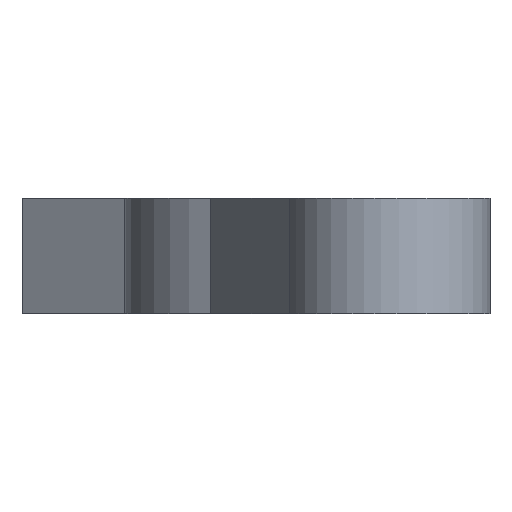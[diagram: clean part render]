
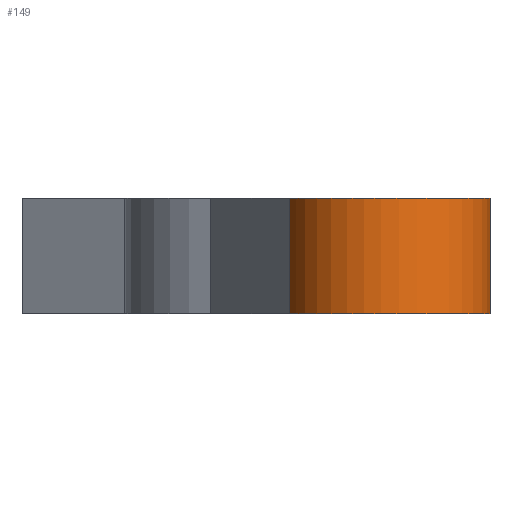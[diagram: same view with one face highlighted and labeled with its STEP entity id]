
A CAD part, left-side view. The second image highlights one B-rep face of the part: STEP entity #149.
In plain terms, the highlighted cylindrical face has radius 4.216 mm (diameter 8.433 mm), a partial arc.
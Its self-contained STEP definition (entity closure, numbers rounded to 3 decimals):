
#3 = VECTOR ( 'NONE', #229, 1000. ) ;
#41 = EDGE_LOOP ( 'NONE', ( #305, #256, #509, #240 ) ) ;
#48 = CIRCLE ( 'NONE', #468, 4.216 ) ;
#68 = DIRECTION ( 'NONE',  ( 1., 0., 0. ) ) ;
#91 = LINE ( 'NONE', #261, #3 ) ;
#96 = LINE ( 'NONE', #133, #669 ) ;
#127 = CARTESIAN_POINT ( 'NONE',  ( 97.778, 23.491, -10.65 ) ) ;
#133 = CARTESIAN_POINT ( 'NONE',  ( 100.156, 15.4, -10.65 ) ) ;
#149 = ADVANCED_FACE ( 'NONE', ( #674 ), #379, .T. ) ;
#167 = DIRECTION ( 'NONE',  ( 0., 0., 1. ) ) ;
#211 = VERTEX_POINT ( 'NONE', #606 ) ;
#222 = CARTESIAN_POINT ( 'NONE',  ( 100.156, 15.4, -10.65 ) ) ;
#229 = DIRECTION ( 'NONE',  ( 0., 0., 1. ) ) ;
#240 = ORIENTED_EDGE ( 'NONE', *, *, #474, .T. ) ;
#256 = ORIENTED_EDGE ( 'NONE', *, *, #407, .F. ) ;
#261 = CARTESIAN_POINT ( 'NONE',  ( 97.778, 23.491, -10.65 ) ) ;
#275 = EDGE_CURVE ( 'NONE', #470, #414, #473, .T. ) ;
#282 = CARTESIAN_POINT ( 'NONE',  ( 97.778, 23.491, -5.9 ) ) ;
#305 = ORIENTED_EDGE ( 'NONE', *, *, #343, .F. ) ;
#323 = DIRECTION ( 'NONE',  ( 0., 0., 1. ) ) ;
#343 = EDGE_CURVE ( 'NONE', #402, #211, #48, .T. ) ;
#379 = CYLINDRICAL_SURFACE ( 'NONE', #582, 4.216 ) ;
#402 = VERTEX_POINT ( 'NONE', #282 ) ;
#407 = EDGE_CURVE ( 'NONE', #470, #402, #91, .T. ) ;
#414 = VERTEX_POINT ( 'NONE', #222 ) ;
#430 = DIRECTION ( 'NONE',  ( 1., 0., 0. ) ) ;
#435 = DIRECTION ( 'NONE',  ( 0., 0., 1. ) ) ;
#437 = CARTESIAN_POINT ( 'NONE',  ( 98.967, 19.446, -10.65 ) ) ;
#468 = AXIS2_PLACEMENT_3D ( 'NONE', #563, #554, #495 ) ;
#470 = VERTEX_POINT ( 'NONE', #127 ) ;
#473 = CIRCLE ( 'NONE', #524, 4.216 ) ;
#474 = EDGE_CURVE ( 'NONE', #414, #211, #96, .T. ) ;
#495 = DIRECTION ( 'NONE',  ( 1., 0., 0. ) ) ;
#509 = ORIENTED_EDGE ( 'NONE', *, *, #275, .T. ) ;
#524 = AXIS2_PLACEMENT_3D ( 'NONE', #437, #435, #430 ) ;
#554 = DIRECTION ( 'NONE',  ( 0., 0., 1. ) ) ;
#563 = CARTESIAN_POINT ( 'NONE',  ( 98.967, 19.446, -5.9 ) ) ;
#582 = AXIS2_PLACEMENT_3D ( 'NONE', #601, #323, #68 ) ;
#601 = CARTESIAN_POINT ( 'NONE',  ( 98.967, 19.446, -10.65 ) ) ;
#606 = CARTESIAN_POINT ( 'NONE',  ( 100.156, 15.4, -5.9 ) ) ;
#669 = VECTOR ( 'NONE', #167, 1000. ) ;
#674 = FACE_OUTER_BOUND ( 'NONE', #41, .T. ) ;
